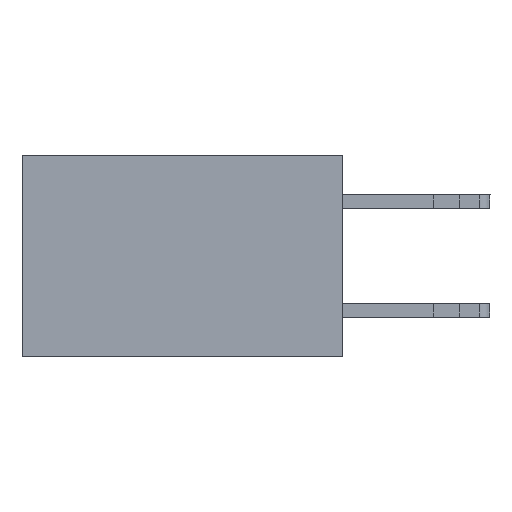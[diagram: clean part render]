
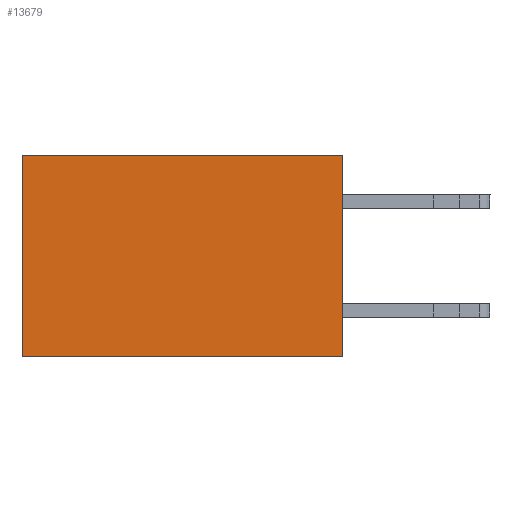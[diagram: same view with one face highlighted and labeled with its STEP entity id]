
A CAD part, left-side view. The second image highlights one B-rep face of the part: STEP entity #13679.
In plain terms, the highlighted planar face has unit normal (-1, 0, 0).
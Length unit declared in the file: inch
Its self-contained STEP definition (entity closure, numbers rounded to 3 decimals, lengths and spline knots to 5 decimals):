
#17 = ORIENTED_EDGE ( 'NONE', *, *, #15073, .T. ) ;
#447 = DIRECTION ( 'NONE',  ( 0., 0., -1. ) ) ;
#720 = ORIENTED_EDGE ( 'NONE', *, *, #11771, .F. ) ;
#1596 = DIRECTION ( 'NONE',  ( 0., 0., -1. ) ) ;
#2540 = LINE ( 'NONE', #4115, #4079 ) ;
#2885 = DIRECTION ( 'NONE',  ( 0., 1., 0. ) ) ;
#3036 = CARTESIAN_POINT ( 'NONE',  ( 0.277, 0.59, 0. ) ) ;
#3305 = CARTESIAN_POINT ( 'NONE',  ( 0.277, 0., -0.37 ) ) ;
#3561 = VERTEX_POINT ( 'NONE', #13435 ) ;
#3643 = CARTESIAN_POINT ( 'NONE',  ( 0.277, 0., -0.37 ) ) ;
#4079 = VECTOR ( 'NONE', #2885, 39.37008 ) ;
#4115 = CARTESIAN_POINT ( 'NONE',  ( 0.277, 0., 0. ) ) ;
#4448 = CARTESIAN_POINT ( 'NONE',  ( 0.277, 0.59, -0.37 ) ) ;
#5922 = EDGE_CURVE ( 'NONE', #10929, #12830, #12291, .T. ) ;
#6371 = PLANE ( 'NONE',  #7121 ) ;
#7121 = AXIS2_PLACEMENT_3D ( 'NONE', #14356, #11712, #17071 ) ;
#8019 = ORIENTED_EDGE ( 'NONE', *, *, #9017, .F. ) ;
#8416 = CARTESIAN_POINT ( 'NONE',  ( 0.277, 0.59, -0.37 ) ) ;
#8684 = VECTOR ( 'NONE', #9088, 39.37008 ) ;
#9017 = EDGE_CURVE ( 'NONE', #14143, #3561, #16841, .T. ) ;
#9088 = DIRECTION ( 'NONE',  ( 0., 1., 0. ) ) ;
#10536 = EDGE_LOOP ( 'NONE', ( #17113, #720, #8019, #17 ) ) ;
#10929 = VERTEX_POINT ( 'NONE', #3036 ) ;
#11628 = FACE_OUTER_BOUND ( 'NONE', #10536, .T. ) ;
#11712 = DIRECTION ( 'NONE',  ( 1., 0., 0. ) ) ;
#11771 = EDGE_CURVE ( 'NONE', #3561, #12830, #16992, .T. ) ;
#12023 = VECTOR ( 'NONE', #1596, 39.37008 ) ;
#12291 = LINE ( 'NONE', #8416, #12023 ) ;
#12830 = VERTEX_POINT ( 'NONE', #4448 ) ;
#13316 = CARTESIAN_POINT ( 'NONE',  ( 0.277, 0., 0. ) ) ;
#13435 = CARTESIAN_POINT ( 'NONE',  ( 0.277, 0., -0.37 ) ) ;
#13679 = ADVANCED_FACE ( 'NONE', ( #11628 ), #6371, .F. ) ;
#14143 = VERTEX_POINT ( 'NONE', #13316 ) ;
#14356 = CARTESIAN_POINT ( 'NONE',  ( 0.277, 0., -0.37 ) ) ;
#14456 = VECTOR ( 'NONE', #447, 39.37008 ) ;
#15073 = EDGE_CURVE ( 'NONE', #14143, #10929, #2540, .T. ) ;
#16841 = LINE ( 'NONE', #3305, #14456 ) ;
#16992 = LINE ( 'NONE', #3643, #8684 ) ;
#17071 = DIRECTION ( 'NONE',  ( 0., 0., -1. ) ) ;
#17113 = ORIENTED_EDGE ( 'NONE', *, *, #5922, .T. ) ;
